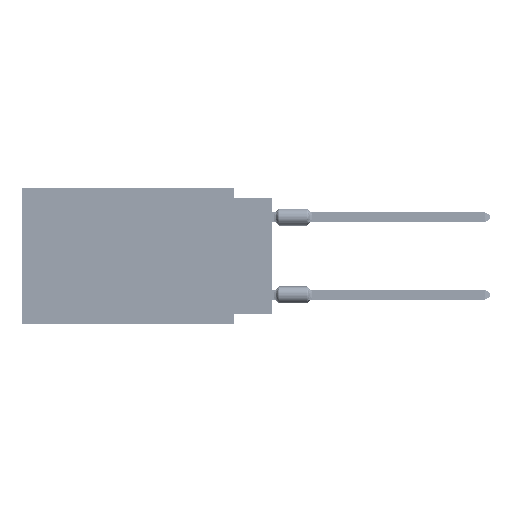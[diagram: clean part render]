
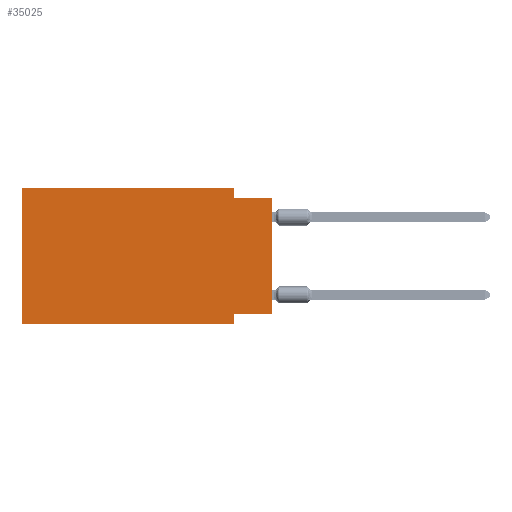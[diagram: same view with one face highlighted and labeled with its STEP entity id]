
A CAD part, left-side view. The second image highlights one B-rep face of the part: STEP entity #35025.
In plain terms, the highlighted planar face has unit normal (-1, 0, 0).
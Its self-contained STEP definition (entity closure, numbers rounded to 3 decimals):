
#2558 = AXIS2_PLACEMENT_3D ( 'NONE', #65541, #9710, #16032 ) ;
#3094 = EDGE_CURVE ( 'NONE', #43083, #48130, #25361, .T. ) ;
#3124 = VERTEX_POINT ( 'NONE', #30380 ) ;
#3370 = LINE ( 'NONE', #42497, #10069 ) ;
#3794 = LINE ( 'NONE', #45229, #47810 ) ;
#4371 = PLANE ( 'NONE',  #2558 ) ;
#5236 = ORIENTED_EDGE ( 'NONE', *, *, #49967, .F. ) ;
#5306 = DIRECTION ( 'NONE',  ( 0., 0., -1. ) ) ;
#5753 = ORIENTED_EDGE ( 'NONE', *, *, #36822, .F. ) ;
#6363 = CARTESIAN_POINT ( 'NONE',  ( 0., 2.54, -0.635 ) ) ;
#9634 = VERTEX_POINT ( 'NONE', #24218 ) ;
#9710 = DIRECTION ( 'NONE',  ( 1., 0., 0. ) ) ;
#10069 = VECTOR ( 'NONE', #63866, 1000. ) ;
#10337 = LINE ( 'NONE', #51132, #44244 ) ;
#10714 = EDGE_CURVE ( 'NONE', #23647, #43083, #10337, .T. ) ;
#11077 = LINE ( 'NONE', #41504, #65680 ) ;
#11419 = VECTOR ( 'NONE', #41465, 1000. ) ;
#12147 = EDGE_CURVE ( 'NONE', #49282, #29285, #3370, .T. ) ;
#12428 = ORIENTED_EDGE ( 'NONE', *, *, #3094, .F. ) ;
#12928 = LINE ( 'NONE', #17596, #36764 ) ;
#16032 = DIRECTION ( 'NONE',  ( 0., 0., -1. ) ) ;
#17188 = VERTEX_POINT ( 'NONE', #63260 ) ;
#17596 = CARTESIAN_POINT ( 'NONE',  ( 0., 16.383, -8.89 ) ) ;
#17823 = CARTESIAN_POINT ( 'NONE',  ( 0., 0., -0.635 ) ) ;
#20258 = VECTOR ( 'NONE', #50097, 1000. ) ;
#23647 = VERTEX_POINT ( 'NONE', #47476 ) ;
#24008 = CARTESIAN_POINT ( 'NONE',  ( 0., 16.383, 0. ) ) ;
#24218 = CARTESIAN_POINT ( 'NONE',  ( 0., 0., -8.255 ) ) ;
#24521 = LINE ( 'NONE', #42123, #11419 ) ;
#25361 = LINE ( 'NONE', #30703, #42461 ) ;
#25481 = ORIENTED_EDGE ( 'NONE', *, *, #47067, .T. ) ;
#27324 = CARTESIAN_POINT ( 'NONE',  ( 0., 2.54, -8.89 ) ) ;
#29285 = VERTEX_POINT ( 'NONE', #27324 ) ;
#30380 = CARTESIAN_POINT ( 'NONE',  ( 0., 16.383, 0. ) ) ;
#30703 = CARTESIAN_POINT ( 'NONE',  ( 0., 0., -0.635 ) ) ;
#31449 = DIRECTION ( 'NONE',  ( 0., 1., 0. ) ) ;
#32611 = EDGE_LOOP ( 'NONE', ( #59964, #12428, #50917, #5236, #42620, #25481, #47085, #5753 ) ) ;
#35025 = ADVANCED_FACE ( 'NONE', ( #50190 ), #4371, .F. ) ;
#35678 = LINE ( 'NONE', #24008, #20258 ) ;
#36764 = VECTOR ( 'NONE', #38013, 1000. ) ;
#36822 = EDGE_CURVE ( 'NONE', #9634, #49282, #11077, .T. ) ;
#38013 = DIRECTION ( 'NONE',  ( 0., -1., 0. ) ) ;
#41465 = DIRECTION ( 'NONE',  ( 0., -1., 0. ) ) ;
#41504 = CARTESIAN_POINT ( 'NONE',  ( 0., 0., -8.255 ) ) ;
#42123 = CARTESIAN_POINT ( 'NONE',  ( 0., 16.383, 0. ) ) ;
#42461 = VECTOR ( 'NONE', #47081, 1000. ) ;
#42497 = CARTESIAN_POINT ( 'NONE',  ( 0., 2.54, -8.89 ) ) ;
#42620 = ORIENTED_EDGE ( 'NONE', *, *, #57991, .F. ) ;
#43083 = VERTEX_POINT ( 'NONE', #6363 ) ;
#44244 = VECTOR ( 'NONE', #5306, 1000. ) ;
#45229 = CARTESIAN_POINT ( 'NONE',  ( 0., 0., 0. ) ) ;
#47067 = EDGE_CURVE ( 'NONE', #17188, #29285, #12928, .T. ) ;
#47081 = DIRECTION ( 'NONE',  ( 0., -1., 0. ) ) ;
#47085 = ORIENTED_EDGE ( 'NONE', *, *, #12147, .F. ) ;
#47476 = CARTESIAN_POINT ( 'NONE',  ( 0., 2.54, 0. ) ) ;
#47810 = VECTOR ( 'NONE', #65614, 1000. ) ;
#48130 = VERTEX_POINT ( 'NONE', #17823 ) ;
#49282 = VERTEX_POINT ( 'NONE', #57390 ) ;
#49967 = EDGE_CURVE ( 'NONE', #3124, #23647, #24521, .T. ) ;
#50097 = DIRECTION ( 'NONE',  ( 0., 0., 1. ) ) ;
#50190 = FACE_OUTER_BOUND ( 'NONE', #32611, .T. ) ;
#50917 = ORIENTED_EDGE ( 'NONE', *, *, #10714, .F. ) ;
#51132 = CARTESIAN_POINT ( 'NONE',  ( 0., 2.54, 0. ) ) ;
#57390 = CARTESIAN_POINT ( 'NONE',  ( 0., 2.54, -8.255 ) ) ;
#57991 = EDGE_CURVE ( 'NONE', #17188, #3124, #35678, .T. ) ;
#59964 = ORIENTED_EDGE ( 'NONE', *, *, #61322, .T. ) ;
#61322 = EDGE_CURVE ( 'NONE', #9634, #48130, #3794, .T. ) ;
#63260 = CARTESIAN_POINT ( 'NONE',  ( 0., 16.383, -8.89 ) ) ;
#63866 = DIRECTION ( 'NONE',  ( 0., 0., -1. ) ) ;
#65541 = CARTESIAN_POINT ( 'NONE',  ( 0., 16.383, 0. ) ) ;
#65614 = DIRECTION ( 'NONE',  ( 0., 0., 1. ) ) ;
#65680 = VECTOR ( 'NONE', #31449, 1000. ) ;
